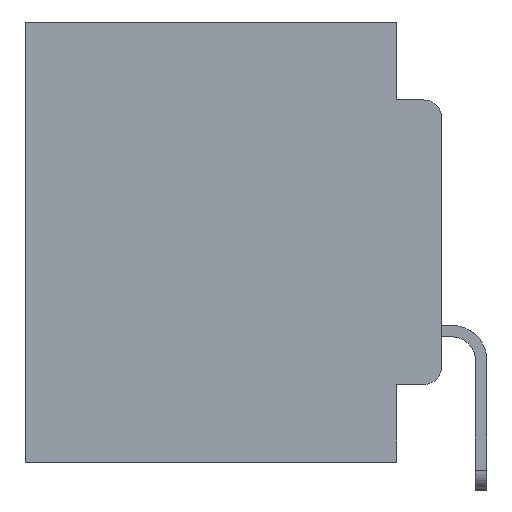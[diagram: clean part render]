
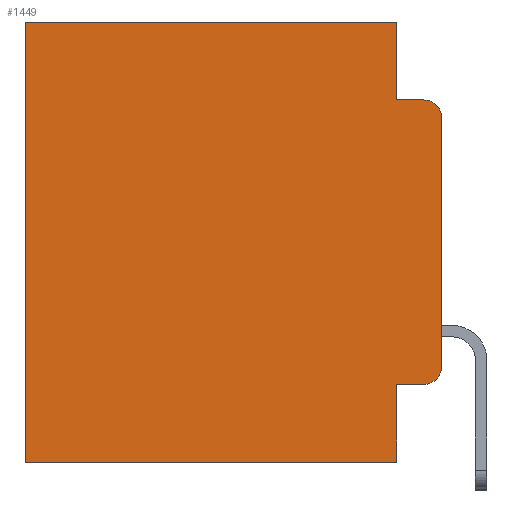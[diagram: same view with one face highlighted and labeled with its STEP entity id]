
A CAD part, left-side view. The second image highlights one B-rep face of the part: STEP entity #1449.
In plain terms, the highlighted planar face has unit normal (-1, 0, 0).
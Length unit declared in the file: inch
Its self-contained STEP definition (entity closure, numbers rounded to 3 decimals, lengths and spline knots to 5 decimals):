
#259 = ORIENTED_EDGE ( 'NONE', *, *, #25943, .T. ) ;
#325 = EDGE_CURVE ( 'NONE', #3272, #17652, #7192, .T. ) ;
#1294 = DIRECTION ( 'NONE',  ( 0., 0., -1. ) ) ;
#1449 = ADVANCED_FACE ( 'NONE', ( #16298 ), #18229, .F. ) ;
#1663 = CARTESIAN_POINT ( 'NONE',  ( 0.298, 0., 0. ) ) ;
#1689 = CARTESIAN_POINT ( 'NONE',  ( 0.298, 0.051, -0.5 ) ) ;
#1858 = VECTOR ( 'NONE', #5255, 39.37008 ) ;
#1986 = AXIS2_PLACEMENT_3D ( 'NONE', #25542, #17938, #3729 ) ;
#2167 = CARTESIAN_POINT ( 'NONE',  ( 0.298, 0.051, -0.4115 ) ) ;
#2206 = VECTOR ( 'NONE', #11859, 39.37008 ) ;
#2552 = CARTESIAN_POINT ( 'NONE',  ( 0.298, 0.02, -0.4115 ) ) ;
#2568 = ORIENTED_EDGE ( 'NONE', *, *, #23518, .F. ) ;
#2702 = AXIS2_PLACEMENT_3D ( 'NONE', #23951, #3800, #10719 ) ;
#2705 = EDGE_CURVE ( 'NONE', #14210, #10395, #23171, .T. ) ;
#3189 = CARTESIAN_POINT ( 'NONE',  ( 0.298, 0.473, 0. ) ) ;
#3272 = VERTEX_POINT ( 'NONE', #1689 ) ;
#3303 = VECTOR ( 'NONE', #1294, 39.37008 ) ;
#3729 = DIRECTION ( 'NONE',  ( 0., 0., -1. ) ) ;
#3785 = AXIS2_PLACEMENT_3D ( 'NONE', #11631, #15706, #19760 ) ;
#3800 = DIRECTION ( 'NONE',  ( 1., 0., 0. ) ) ;
#3898 = ORIENTED_EDGE ( 'NONE', *, *, #24840, .F. ) ;
#4809 = CARTESIAN_POINT ( 'NONE',  ( 0.298, 0.051, 0. ) ) ;
#5255 = DIRECTION ( 'NONE',  ( 0., 1., 0. ) ) ;
#5672 = DIRECTION ( 'NONE',  ( 0., 0., -1. ) ) ;
#5808 = LINE ( 'NONE', #17382, #22034 ) ;
#7192 = LINE ( 'NONE', #9577, #22174 ) ;
#7885 = LINE ( 'NONE', #25749, #1858 ) ;
#9492 = CARTESIAN_POINT ( 'NONE',  ( 0.298, 0.051, 0. ) ) ;
#9503 = CARTESIAN_POINT ( 'NONE',  ( 0.298, 0.02, -0.0885 ) ) ;
#9577 = CARTESIAN_POINT ( 'NONE',  ( 0.298, 0., -0.5 ) ) ;
#9653 = VERTEX_POINT ( 'NONE', #3189 ) ;
#10395 = VERTEX_POINT ( 'NONE', #23751 ) ;
#10719 = DIRECTION ( 'NONE',  ( 0., 0., -1. ) ) ;
#10941 = EDGE_CURVE ( 'NONE', #15441, #21461, #11607, .T. ) ;
#11607 = LINE ( 'NONE', #9492, #3303 ) ;
#11631 = CARTESIAN_POINT ( 'NONE',  ( 0.298, 0.02, -0.1085 ) ) ;
#11859 = DIRECTION ( 'NONE',  ( 0., -1., 0. ) ) ;
#11934 = EDGE_LOOP ( 'NONE', ( #24373, #24806, #2568, #16554, #259, #19611, #24337, #3898, #15770, #15053 ) ) ;
#12344 = DIRECTION ( 'NONE',  ( 0., 0., -1. ) ) ;
#12645 = CARTESIAN_POINT ( 'NONE',  ( 0.298, 0.473, 0. ) ) ;
#13085 = CIRCLE ( 'NONE', #1986, 0.02 ) ;
#13941 = EDGE_CURVE ( 'NONE', #9653, #17652, #24592, .T. ) ;
#14210 = VERTEX_POINT ( 'NONE', #22954 ) ;
#15053 = ORIENTED_EDGE ( 'NONE', *, *, #15960, .T. ) ;
#15117 = VECTOR ( 'NONE', #24433, 39.37008 ) ;
#15380 = VERTEX_POINT ( 'NONE', #2167 ) ;
#15441 = VERTEX_POINT ( 'NONE', #4809 ) ;
#15706 = DIRECTION ( 'NONE',  ( -1., 0., 0. ) ) ;
#15770 = ORIENTED_EDGE ( 'NONE', *, *, #16797, .T. ) ;
#15960 = EDGE_CURVE ( 'NONE', #22762, #10395, #13085, .T. ) ;
#16298 = FACE_OUTER_BOUND ( 'NONE', #11934, .T. ) ;
#16527 = LINE ( 'NONE', #22459, #22262 ) ;
#16554 = ORIENTED_EDGE ( 'NONE', *, *, #10941, .F. ) ;
#16797 = EDGE_CURVE ( 'NONE', #15380, #22762, #25059, .T. ) ;
#17382 = CARTESIAN_POINT ( 'NONE',  ( 0.298, 0.051, -0.0885 ) ) ;
#17652 = VERTEX_POINT ( 'NONE', #23122 ) ;
#17938 = DIRECTION ( 'NONE',  ( -1., 0., 0. ) ) ;
#18229 = PLANE ( 'NONE',  #2702 ) ;
#19611 = ORIENTED_EDGE ( 'NONE', *, *, #13941, .T. ) ;
#19760 = DIRECTION ( 'NONE',  ( 0., 0., -1. ) ) ;
#19764 = DIRECTION ( 'NONE',  ( 0., 1., 0. ) ) ;
#20879 = EDGE_CURVE ( 'NONE', #14210, #21878, #22458, .T. ) ;
#21461 = VERTEX_POINT ( 'NONE', #22555 ) ;
#21878 = VERTEX_POINT ( 'NONE', #9503 ) ;
#22034 = VECTOR ( 'NONE', #22799, 39.37008 ) ;
#22174 = VECTOR ( 'NONE', #19764, 39.37008 ) ;
#22262 = VECTOR ( 'NONE', #12344, 39.37008 ) ;
#22458 = CIRCLE ( 'NONE', #3785, 0.02 ) ;
#22459 = CARTESIAN_POINT ( 'NONE',  ( 0.298, 0.051, 0. ) ) ;
#22555 = CARTESIAN_POINT ( 'NONE',  ( 0.298, 0.051, -0.0885 ) ) ;
#22762 = VERTEX_POINT ( 'NONE', #2552 ) ;
#22799 = DIRECTION ( 'NONE',  ( 0., -1., 0. ) ) ;
#22954 = CARTESIAN_POINT ( 'NONE',  ( 0.298, 0., -0.1085 ) ) ;
#23122 = CARTESIAN_POINT ( 'NONE',  ( 0.298, 0.473, -0.5 ) ) ;
#23171 = LINE ( 'NONE', #1663, #25728 ) ;
#23518 = EDGE_CURVE ( 'NONE', #21461, #21878, #5808, .T. ) ;
#23751 = CARTESIAN_POINT ( 'NONE',  ( 0.298, 0., -0.3915 ) ) ;
#23951 = CARTESIAN_POINT ( 'NONE',  ( 0.298, 0., 0. ) ) ;
#24156 = CARTESIAN_POINT ( 'NONE',  ( 0.298, 0.051, -0.4115 ) ) ;
#24337 = ORIENTED_EDGE ( 'NONE', *, *, #325, .F. ) ;
#24373 = ORIENTED_EDGE ( 'NONE', *, *, #2705, .F. ) ;
#24433 = DIRECTION ( 'NONE',  ( 0., 0., -1. ) ) ;
#24592 = LINE ( 'NONE', #12645, #15117 ) ;
#24806 = ORIENTED_EDGE ( 'NONE', *, *, #20879, .T. ) ;
#24840 = EDGE_CURVE ( 'NONE', #15380, #3272, #16527, .T. ) ;
#25059 = LINE ( 'NONE', #24156, #2206 ) ;
#25542 = CARTESIAN_POINT ( 'NONE',  ( 0.298, 0.02, -0.3915 ) ) ;
#25728 = VECTOR ( 'NONE', #5672, 39.37008 ) ;
#25749 = CARTESIAN_POINT ( 'NONE',  ( 0.298, 0., 0. ) ) ;
#25943 = EDGE_CURVE ( 'NONE', #15441, #9653, #7885, .T. ) ;
